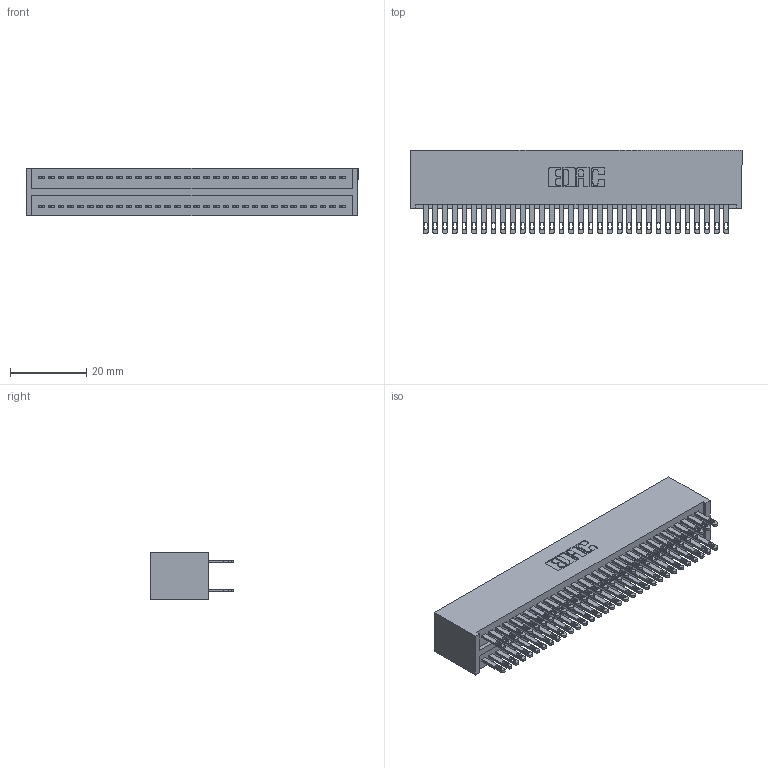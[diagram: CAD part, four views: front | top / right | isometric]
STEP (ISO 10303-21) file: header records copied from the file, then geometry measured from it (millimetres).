
FILE_DESCRIPTION (( 'STEP AP203' ), '1' );
FILE_NAME ('325-064-500-201.STEP', '2020-02-25T03:04:53', ( '' ), ( '' ), 'SwSTEP 2.0', 'SolidWorks 2016', '' );
FILE_SCHEMA (( 'CONFIG_CONTROL_DESIGN' ));
Length unit declared in the file: inch
Products named in the file (3): 325 Part_Lugless; 325-292-001_325-293-100; 325-064-500-201
Assembly tree (65 placements, depth 2):
  325-064-500-201
    325 Part_Lugless
    325-292-001_325-293-100  x64
Bounding box: 86.92 x 21.84 x 12.45 mm (x, y, z)
Volume: 11932.8 mm3; surface area: 15536.2 mm2
Topology: 65 solids, 65 shells, 3178 faces, 9695 edges, 6462 vertices
Faces by surface type: plane 1986, cylinder 1192
Entity records: 21533 total; most frequent: CARTESIAN_POINT 3578, ORIENTED_EDGE 3514, DIRECTION 3069, EDGE_CURVE 1757, VECTOR 1633, LINE 1633, VERTEX_POINT 1170, AXIS2_PLACEMENT_3D 718
